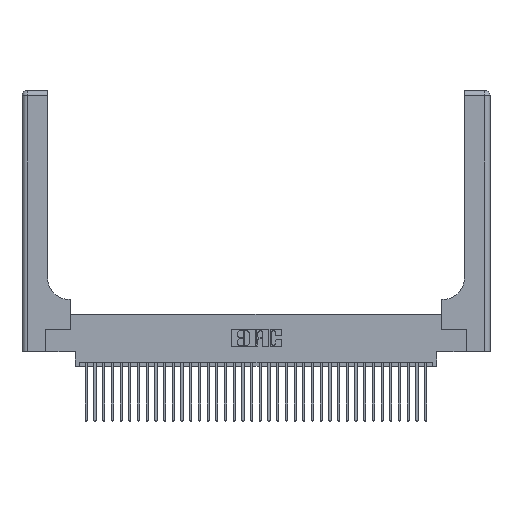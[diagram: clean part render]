
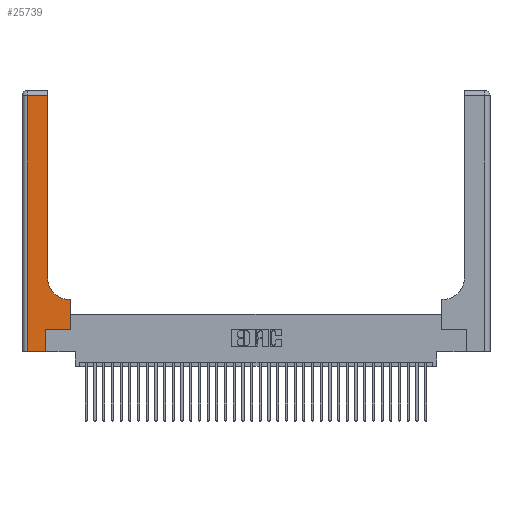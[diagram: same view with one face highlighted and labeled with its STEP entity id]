
A CAD part, top view. The second image highlights one B-rep face of the part: STEP entity #25739.
In plain terms, the highlighted planar face has unit normal (0, 0, 1).
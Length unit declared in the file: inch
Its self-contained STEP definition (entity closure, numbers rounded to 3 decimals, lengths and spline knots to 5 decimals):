
#3 = LINE ( 'NONE', #35140, #35235 ) ;
#86 = CARTESIAN_POINT ( 'NONE',  ( 0.2915, 3., 0.37 ) ) ;
#183 = CARTESIAN_POINT ( 'NONE',  ( 0.269, 0.25, 0.37 ) ) ;
#223 = ORIENTED_EDGE ( 'NONE', *, *, #15647, .T. ) ;
#605 = VERTEX_POINT ( 'NONE', #16859 ) ;
#618 = DIRECTION ( 'NONE',  ( 1., 0., 0. ) ) ;
#909 = CARTESIAN_POINT ( 'NONE',  ( 0.06, 3., 0.37 ) ) ;
#965 = VECTOR ( 'NONE', #30539, 39.37008 ) ;
#1157 = VECTOR ( 'NONE', #1951, 39.37008 ) ;
#1174 = DIRECTION ( 'NONE',  ( 0., -1., 0. ) ) ;
#1886 = CARTESIAN_POINT ( 'NONE',  ( 0.2915, 2.94, 0.37 ) ) ;
#1951 = DIRECTION ( 'NONE',  ( 0., 1., 0. ) ) ;
#2956 = LINE ( 'NONE', #25560, #20331 ) ;
#3193 = ORIENTED_EDGE ( 'NONE', *, *, #26568, .T. ) ;
#3307 = LINE ( 'NONE', #909, #19879 ) ;
#5326 = VERTEX_POINT ( 'NONE', #1886 ) ;
#5987 = CARTESIAN_POINT ( 'NONE',  ( 0.5415, 0.6, 0.37 ) ) ;
#6209 = CARTESIAN_POINT ( 'NONE',  ( 0., 2.94, 0.37 ) ) ;
#6346 = ORIENTED_EDGE ( 'NONE', *, *, #32002, .T. ) ;
#6727 = EDGE_CURVE ( 'NONE', #14958, #605, #20269, .T. ) ;
#7013 = VECTOR ( 'NONE', #22692, 39.37008 ) ;
#7573 = CARTESIAN_POINT ( 'NONE',  ( 0., 0., 0.37 ) ) ;
#8855 = LINE ( 'NONE', #183, #11955 ) ;
#9987 = ORIENTED_EDGE ( 'NONE', *, *, #6727, .T. ) ;
#10522 = PLANE ( 'NONE',  #21399 ) ;
#11355 = DIRECTION ( 'NONE',  ( 1., 0., 0. ) ) ;
#11955 = VECTOR ( 'NONE', #11355, 39.37008 ) ;
#11956 = LINE ( 'NONE', #27656, #1157 ) ;
#14198 = EDGE_LOOP ( 'NONE', ( #3193, #34541, #223, #9987, #35818, #33762, #6346, #30015, #36009 ) ) ;
#14958 = VERTEX_POINT ( 'NONE', #32305 ) ;
#15647 = EDGE_CURVE ( 'NONE', #17967, #14958, #3307, .T. ) ;
#16160 = LINE ( 'NONE', #6209, #21466 ) ;
#16750 = VERTEX_POINT ( 'NONE', #26261 ) ;
#16859 = CARTESIAN_POINT ( 'NONE',  ( 0.269, 0., 0.37 ) ) ;
#17458 = FACE_OUTER_BOUND ( 'NONE', #14198, .T. ) ;
#17967 = VERTEX_POINT ( 'NONE', #33470 ) ;
#19877 = EDGE_CURVE ( 'NONE', #605, #34977, #11956, .T. ) ;
#19879 = VECTOR ( 'NONE', #1174, 39.37008 ) ;
#20269 = LINE ( 'NONE', #7573, #965 ) ;
#20331 = VECTOR ( 'NONE', #31190, 39.37008 ) ;
#20414 = CARTESIAN_POINT ( 'NONE',  ( 0.5415, 0.85, 0.37 ) ) ;
#20423 = LINE ( 'NONE', #86, #7013 ) ;
#20458 = DIRECTION ( 'NONE',  ( -1., 0., 0. ) ) ;
#21173 = AXIS2_PLACEMENT_3D ( 'NONE', #20414, #31990, #618 ) ;
#21399 = AXIS2_PLACEMENT_3D ( 'NONE', #36226, #36371, #22251 ) ;
#21466 = VECTOR ( 'NONE', #20458, 39.37008 ) ;
#22251 = DIRECTION ( 'NONE',  ( -1., 0., 0. ) ) ;
#22692 = DIRECTION ( 'NONE',  ( 0., 1., 0. ) ) ;
#23100 = CIRCLE ( 'NONE', #21173, 0.25 ) ;
#23490 = CARTESIAN_POINT ( 'NONE',  ( 0.5585, 0.6, 0.37 ) ) ;
#24064 = VERTEX_POINT ( 'NONE', #5987 ) ;
#25560 = CARTESIAN_POINT ( 'NONE',  ( 0.5585, 0.25, 0.37 ) ) ;
#25581 = CARTESIAN_POINT ( 'NONE',  ( 0.269, 0.25, 0.37 ) ) ;
#25739 = ADVANCED_FACE ( 'NONE', ( #17458 ), #10522, .F. ) ;
#26261 = CARTESIAN_POINT ( 'NONE',  ( 0.5585, 0.25, 0.37 ) ) ;
#26568 = EDGE_CURVE ( 'NONE', #34984, #5326, #20423, .T. ) ;
#26633 = EDGE_CURVE ( 'NONE', #34977, #16750, #8855, .T. ) ;
#27157 = EDGE_CURVE ( 'NONE', #24064, #34984, #23100, .T. ) ;
#27656 = CARTESIAN_POINT ( 'NONE',  ( 0.269, 0., 0.37 ) ) ;
#27945 = VERTEX_POINT ( 'NONE', #23490 ) ;
#29080 = EDGE_CURVE ( 'NONE', #27945, #24064, #3, .T. ) ;
#30015 = ORIENTED_EDGE ( 'NONE', *, *, #29080, .T. ) ;
#30539 = DIRECTION ( 'NONE',  ( 1., 0., 0. ) ) ;
#31190 = DIRECTION ( 'NONE',  ( 0., 1., 0. ) ) ;
#31207 = CARTESIAN_POINT ( 'NONE',  ( 0.2915, 0.85, 0.37 ) ) ;
#31990 = DIRECTION ( 'NONE',  ( 0., 0., -1. ) ) ;
#32002 = EDGE_CURVE ( 'NONE', #16750, #27945, #2956, .T. ) ;
#32305 = CARTESIAN_POINT ( 'NONE',  ( 0.06, 0., 0.37 ) ) ;
#32365 = DIRECTION ( 'NONE',  ( -1., 0., 0. ) ) ;
#33470 = CARTESIAN_POINT ( 'NONE',  ( 0.06, 2.94, 0.37 ) ) ;
#33762 = ORIENTED_EDGE ( 'NONE', *, *, #26633, .T. ) ;
#34475 = EDGE_CURVE ( 'NONE', #5326, #17967, #16160, .T. ) ;
#34541 = ORIENTED_EDGE ( 'NONE', *, *, #34475, .T. ) ;
#34977 = VERTEX_POINT ( 'NONE', #25581 ) ;
#34984 = VERTEX_POINT ( 'NONE', #31207 ) ;
#35140 = CARTESIAN_POINT ( 'NONE',  ( 0.2915, 0.6, 0.37 ) ) ;
#35235 = VECTOR ( 'NONE', #32365, 39.37008 ) ;
#35818 = ORIENTED_EDGE ( 'NONE', *, *, #19877, .T. ) ;
#36009 = ORIENTED_EDGE ( 'NONE', *, *, #27157, .T. ) ;
#36226 = CARTESIAN_POINT ( 'NONE',  ( 0., 3., 0.37 ) ) ;
#36371 = DIRECTION ( 'NONE',  ( 0., 0., -1. ) ) ;
